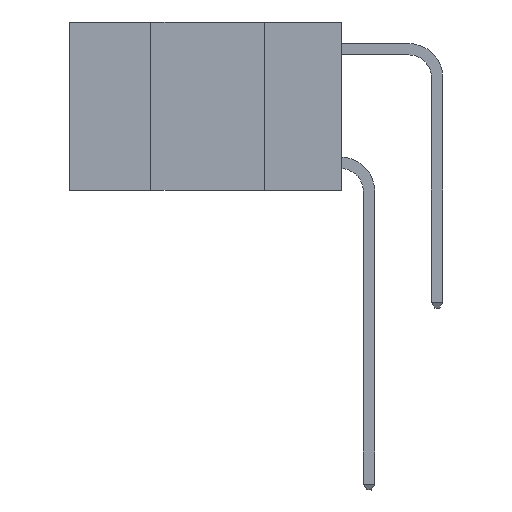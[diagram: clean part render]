
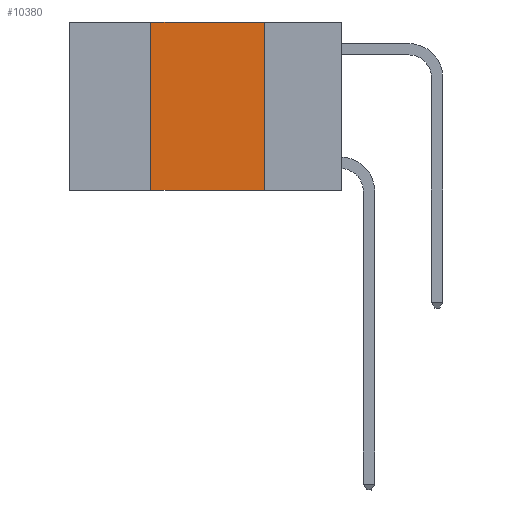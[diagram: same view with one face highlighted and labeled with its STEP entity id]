
A CAD part, left-side view. The second image highlights one B-rep face of the part: STEP entity #10380.
In plain terms, the highlighted planar face has unit normal (-1, 0, 0).
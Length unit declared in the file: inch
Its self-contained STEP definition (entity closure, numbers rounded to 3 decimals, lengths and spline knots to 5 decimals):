
#205 = VERTEX_POINT ( 'NONE', #16963 ) ;
#290 = CARTESIAN_POINT ( 'NONE',  ( 0., 0.42, 0. ) ) ;
#1001 = ORIENTED_EDGE ( 'NONE', *, *, #1039, .T. ) ;
#1039 = EDGE_CURVE ( 'NONE', #17625, #2149, #25172, .T. ) ;
#1316 = CARTESIAN_POINT ( 'NONE',  ( 0., 0.6, -0.37 ) ) ;
#1377 = CARTESIAN_POINT ( 'NONE',  ( 0., 0.6, 0. ) ) ;
#1998 = AXIS2_PLACEMENT_3D ( 'NONE', #1377, #3562, #18666 ) ;
#2149 = VERTEX_POINT ( 'NONE', #9973 ) ;
#2283 = EDGE_LOOP ( 'NONE', ( #12831, #27557, #16247, #1001 ) ) ;
#2299 = VECTOR ( 'NONE', #23710, 39.37008 ) ;
#2508 = EDGE_CURVE ( 'NONE', #17625, #22924, #17439, .T. ) ;
#3562 = DIRECTION ( 'NONE',  ( 1., 0., 0. ) ) ;
#6860 = EDGE_CURVE ( 'NONE', #205, #2149, #24186, .T. ) ;
#8756 = VECTOR ( 'NONE', #16231, 39.37008 ) ;
#8954 = DIRECTION ( 'NONE',  ( 0., 0., -1. ) ) ;
#9973 = CARTESIAN_POINT ( 'NONE',  ( 0., 0.17, -0.37 ) ) ;
#10380 = ADVANCED_FACE ( 'NONE', ( #22668 ), #27120, .F. ) ;
#11188 = DIRECTION ( 'NONE',  ( 0., 0., 1. ) ) ;
#11704 = VECTOR ( 'NONE', #11188, 39.37008 ) ;
#12831 = ORIENTED_EDGE ( 'NONE', *, *, #6860, .F. ) ;
#15187 = LINE ( 'NONE', #18371, #8756 ) ;
#16231 = DIRECTION ( 'NONE',  ( 0., -1., 0. ) ) ;
#16247 = ORIENTED_EDGE ( 'NONE', *, *, #2508, .F. ) ;
#16857 = EDGE_CURVE ( 'NONE', #22924, #205, #15187, .T. ) ;
#16963 = CARTESIAN_POINT ( 'NONE',  ( 0., 0.17, 0. ) ) ;
#17439 = LINE ( 'NONE', #290, #11704 ) ;
#17625 = VERTEX_POINT ( 'NONE', #27261 ) ;
#17877 = VECTOR ( 'NONE', #8954, 39.37008 ) ;
#18371 = CARTESIAN_POINT ( 'NONE',  ( 0., 0.6, 0. ) ) ;
#18666 = DIRECTION ( 'NONE',  ( 0., 0., -1. ) ) ;
#19681 = CARTESIAN_POINT ( 'NONE',  ( 0., 0.17, 0. ) ) ;
#21895 = CARTESIAN_POINT ( 'NONE',  ( 0., 0.42, 0. ) ) ;
#22668 = FACE_OUTER_BOUND ( 'NONE', #2283, .T. ) ;
#22924 = VERTEX_POINT ( 'NONE', #21895 ) ;
#23710 = DIRECTION ( 'NONE',  ( 0., -1., 0. ) ) ;
#24186 = LINE ( 'NONE', #19681, #17877 ) ;
#25172 = LINE ( 'NONE', #1316, #2299 ) ;
#27120 = PLANE ( 'NONE',  #1998 ) ;
#27261 = CARTESIAN_POINT ( 'NONE',  ( 0., 0.42, -0.37 ) ) ;
#27557 = ORIENTED_EDGE ( 'NONE', *, *, #16857, .F. ) ;
